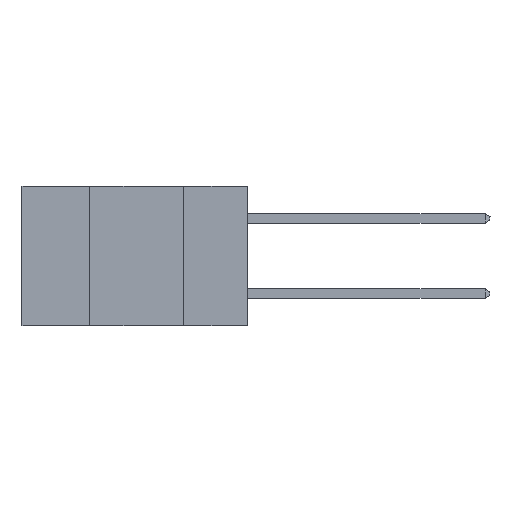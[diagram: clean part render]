
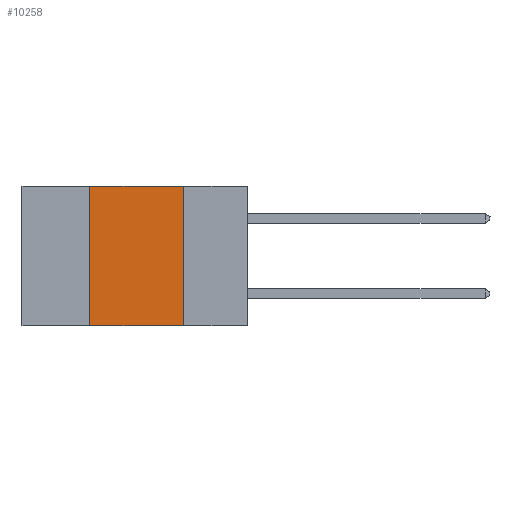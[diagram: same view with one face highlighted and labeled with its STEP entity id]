
A CAD part, left-side view. The second image highlights one B-rep face of the part: STEP entity #10258.
In plain terms, the highlighted planar face has unit normal (-1, 0, 0).
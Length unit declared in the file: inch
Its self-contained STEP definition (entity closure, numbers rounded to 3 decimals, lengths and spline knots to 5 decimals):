
#226 = VERTEX_POINT ( 'NONE', #6619 ) ;
#339 = LINE ( 'NONE', #11015, #6494 ) ;
#749 = CARTESIAN_POINT ( 'NONE',  ( 0., 0.6, -0.37 ) ) ;
#908 = VERTEX_POINT ( 'NONE', #4311 ) ;
#1401 = VECTOR ( 'NONE', #3789, 39.37008 ) ;
#2376 = CARTESIAN_POINT ( 'NONE',  ( 0., 0.42, -0.37 ) ) ;
#2482 = EDGE_LOOP ( 'NONE', ( #9257, #7707, #4072, #11608 ) ) ;
#2808 = EDGE_CURVE ( 'NONE', #12534, #908, #339, .T. ) ;
#3350 = PLANE ( 'NONE',  #4069 ) ;
#3611 = LINE ( 'NONE', #12625, #1401 ) ;
#3789 = DIRECTION ( 'NONE',  ( 0., -1., 0. ) ) ;
#4069 = AXIS2_PLACEMENT_3D ( 'NONE', #9349, #9159, #5210 ) ;
#4072 = ORIENTED_EDGE ( 'NONE', *, *, #6567, .F. ) ;
#4311 = CARTESIAN_POINT ( 'NONE',  ( 0., 0.17, -0.37 ) ) ;
#4579 = LINE ( 'NONE', #5546, #6464 ) ;
#5112 = VERTEX_POINT ( 'NONE', #2376 ) ;
#5210 = DIRECTION ( 'NONE',  ( 0., 0., -1. ) ) ;
#5249 = EDGE_CURVE ( 'NONE', #5112, #908, #8770, .T. ) ;
#5546 = CARTESIAN_POINT ( 'NONE',  ( 0., 0.42, -0.37 ) ) ;
#6182 = VECTOR ( 'NONE', #12616, 39.37008 ) ;
#6464 = VECTOR ( 'NONE', #7354, 39.37008 ) ;
#6494 = VECTOR ( 'NONE', #8180, 39.37008 ) ;
#6567 = EDGE_CURVE ( 'NONE', #5112, #226, #4579, .T. ) ;
#6619 = CARTESIAN_POINT ( 'NONE',  ( 0., 0.42, 0. ) ) ;
#7354 = DIRECTION ( 'NONE',  ( 0., 0., 1. ) ) ;
#7675 = CARTESIAN_POINT ( 'NONE',  ( 0., 0.17, 0. ) ) ;
#7707 = ORIENTED_EDGE ( 'NONE', *, *, #9998, .F. ) ;
#8180 = DIRECTION ( 'NONE',  ( 0., 0., -1. ) ) ;
#8391 = FACE_OUTER_BOUND ( 'NONE', #2482, .T. ) ;
#8770 = LINE ( 'NONE', #749, #6182 ) ;
#9159 = DIRECTION ( 'NONE',  ( 1., 0., 0. ) ) ;
#9257 = ORIENTED_EDGE ( 'NONE', *, *, #2808, .F. ) ;
#9349 = CARTESIAN_POINT ( 'NONE',  ( 0., 0.6, 0. ) ) ;
#9998 = EDGE_CURVE ( 'NONE', #226, #12534, #3611, .T. ) ;
#10258 = ADVANCED_FACE ( 'NONE', ( #8391 ), #3350, .F. ) ;
#11015 = CARTESIAN_POINT ( 'NONE',  ( 0., 0.17, -0.37 ) ) ;
#11608 = ORIENTED_EDGE ( 'NONE', *, *, #5249, .T. ) ;
#12534 = VERTEX_POINT ( 'NONE', #7675 ) ;
#12616 = DIRECTION ( 'NONE',  ( 0., -1., 0. ) ) ;
#12625 = CARTESIAN_POINT ( 'NONE',  ( 0., 0.6, 0. ) ) ;
